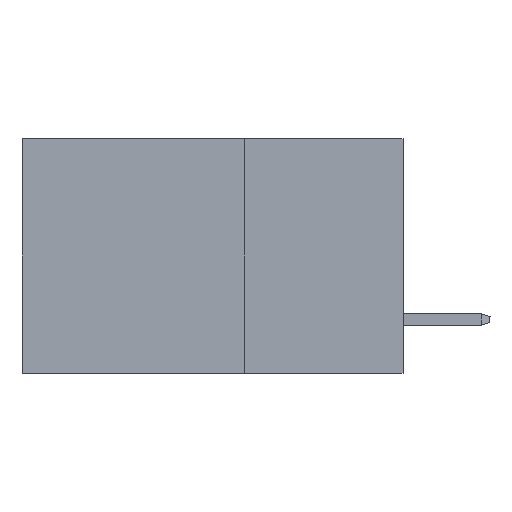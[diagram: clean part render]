
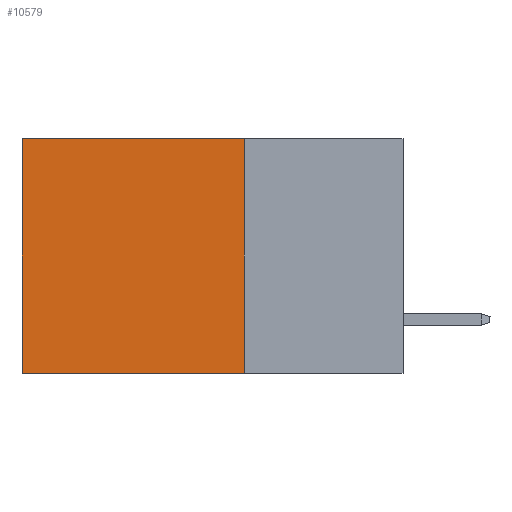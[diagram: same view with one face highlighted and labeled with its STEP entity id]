
A CAD part, left-side view. The second image highlights one B-rep face of the part: STEP entity #10579.
In plain terms, the highlighted planar face has unit normal (-1, 0, 0).
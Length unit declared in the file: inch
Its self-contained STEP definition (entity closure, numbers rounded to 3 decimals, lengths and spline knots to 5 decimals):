
#351 = EDGE_CURVE ( 'NONE', #13703, #12742, #2202, .T. ) ;
#497 = ORIENTED_EDGE ( 'NONE', *, *, #351, .T. ) ;
#507 = LINE ( 'NONE', #5265, #7723 ) ;
#1593 = EDGE_CURVE ( 'NONE', #13703, #8964, #11791, .T. ) ;
#2166 = EDGE_CURVE ( 'NONE', #12742, #13725, #507, .T. ) ;
#2202 = LINE ( 'NONE', #6880, #9384 ) ;
#2536 = DIRECTION ( 'NONE',  ( 0., 1., 0. ) ) ;
#3582 = CARTESIAN_POINT ( 'NONE',  ( 0.2875, 0.25, -0.37 ) ) ;
#3974 = CARTESIAN_POINT ( 'NONE',  ( 0.2875, 0.6, -0.37 ) ) ;
#4030 = DIRECTION ( 'NONE',  ( 1., 0., 0. ) ) ;
#4194 = CARTESIAN_POINT ( 'NONE',  ( 0.2875, 0.25, 0. ) ) ;
#5100 = CARTESIAN_POINT ( 'NONE',  ( 0.2875, 0.25, 0. ) ) ;
#5265 = CARTESIAN_POINT ( 'NONE',  ( 0.2875, 0.6, 0. ) ) ;
#5828 = DIRECTION ( 'NONE',  ( 0., 1., 0. ) ) ;
#5945 = CARTESIAN_POINT ( 'NONE',  ( 0.2875, 0.25, 0. ) ) ;
#6880 = CARTESIAN_POINT ( 'NONE',  ( 0.2875, 0.25, 0. ) ) ;
#7723 = VECTOR ( 'NONE', #9729, 39.37008 ) ;
#8437 = ORIENTED_EDGE ( 'NONE', *, *, #2166, .T. ) ;
#8492 = LINE ( 'NONE', #14030, #9414 ) ;
#8964 = VERTEX_POINT ( 'NONE', #3582 ) ;
#9384 = VECTOR ( 'NONE', #5828, 39.37008 ) ;
#9414 = VECTOR ( 'NONE', #2536, 39.37008 ) ;
#9729 = DIRECTION ( 'NONE',  ( 0., 0., -1. ) ) ;
#9978 = EDGE_LOOP ( 'NONE', ( #8437, #10966, #11506, #497 ) ) ;
#10090 = AXIS2_PLACEMENT_3D ( 'NONE', #5100, #4030, #11920 ) ;
#10395 = VECTOR ( 'NONE', #11718, 39.37008 ) ;
#10579 = ADVANCED_FACE ( 'NONE', ( #12057 ), #13035, .F. ) ;
#10966 = ORIENTED_EDGE ( 'NONE', *, *, #14086, .F. ) ;
#11506 = ORIENTED_EDGE ( 'NONE', *, *, #1593, .F. ) ;
#11718 = DIRECTION ( 'NONE',  ( 0., 0., -1. ) ) ;
#11791 = LINE ( 'NONE', #5945, #10395 ) ;
#11920 = DIRECTION ( 'NONE',  ( 0., 0., -1. ) ) ;
#12057 = FACE_OUTER_BOUND ( 'NONE', #9978, .T. ) ;
#12742 = VERTEX_POINT ( 'NONE', #14942 ) ;
#13035 = PLANE ( 'NONE',  #10090 ) ;
#13703 = VERTEX_POINT ( 'NONE', #4194 ) ;
#13725 = VERTEX_POINT ( 'NONE', #3974 ) ;
#14030 = CARTESIAN_POINT ( 'NONE',  ( 0.2875, 0.25, -0.37 ) ) ;
#14086 = EDGE_CURVE ( 'NONE', #8964, #13725, #8492, .T. ) ;
#14942 = CARTESIAN_POINT ( 'NONE',  ( 0.2875, 0.6, 0. ) ) ;
